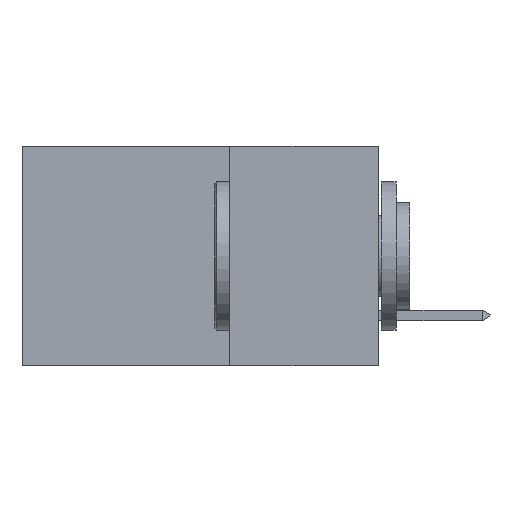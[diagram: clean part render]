
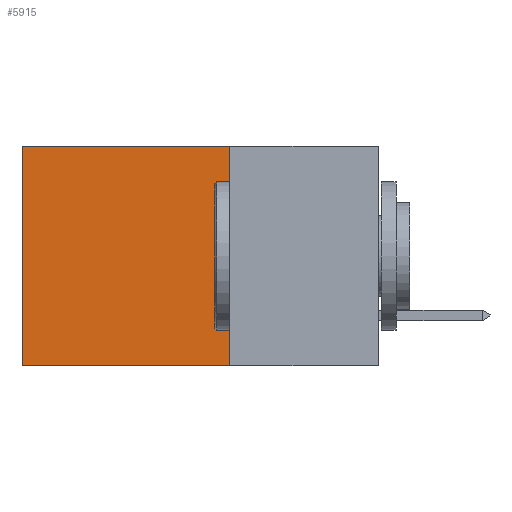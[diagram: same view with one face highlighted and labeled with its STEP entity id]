
A CAD part, left-side view. The second image highlights one B-rep face of the part: STEP entity #5915.
In plain terms, the highlighted planar face has unit normal (-1, 0, 0).
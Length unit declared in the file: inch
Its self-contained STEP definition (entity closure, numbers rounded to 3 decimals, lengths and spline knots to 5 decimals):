
#554 = VERTEX_POINT ( 'NONE', #1012 ) ;
#1012 = CARTESIAN_POINT ( 'NONE',  ( 0.2615, 0.25, -0.37 ) ) ;
#1763 = VERTEX_POINT ( 'NONE', #17823 ) ;
#1865 = EDGE_CURVE ( 'NONE', #14438, #1763, #7289, .T. ) ;
#3894 = CARTESIAN_POINT ( 'NONE',  ( 0.2615, 0.25, 0. ) ) ;
#4946 = CARTESIAN_POINT ( 'NONE',  ( 0.2615, 0.25, -0.37 ) ) ;
#5407 = ORIENTED_EDGE ( 'NONE', *, *, #11227, .F. ) ;
#5505 = CARTESIAN_POINT ( 'NONE',  ( 0.2615, 0.25, -0.37 ) ) ;
#5662 = DIRECTION ( 'NONE',  ( 0., 1., 0. ) ) ;
#5915 = ADVANCED_FACE ( 'NONE', ( #6634 ), #19309, .F. ) ;
#6634 = FACE_OUTER_BOUND ( 'NONE', #19253, .T. ) ;
#7289 = LINE ( 'NONE', #8921, #13518 ) ;
#8307 = VECTOR ( 'NONE', #5662, 39.37008 ) ;
#8531 = DIRECTION ( 'NONE',  ( 0., 1., 0. ) ) ;
#8921 = CARTESIAN_POINT ( 'NONE',  ( 0.2615, 0.25, 0. ) ) ;
#9086 = VECTOR ( 'NONE', #12416, 39.37008 ) ;
#9994 = LINE ( 'NONE', #11817, #8307 ) ;
#10129 = DIRECTION ( 'NONE',  ( 0., 0., -1. ) ) ;
#10196 = VERTEX_POINT ( 'NONE', #11056 ) ;
#10263 = AXIS2_PLACEMENT_3D ( 'NONE', #5505, #12889, #10129 ) ;
#10609 = VECTOR ( 'NONE', #11116, 39.37008 ) ;
#10910 = EDGE_CURVE ( 'NONE', #554, #10196, #9994, .T. ) ;
#11056 = CARTESIAN_POINT ( 'NONE',  ( 0.2615, 0.6, -0.37 ) ) ;
#11092 = CARTESIAN_POINT ( 'NONE',  ( 0.2615, 0.6, -0.37 ) ) ;
#11116 = DIRECTION ( 'NONE',  ( 0., 0., -1. ) ) ;
#11227 = EDGE_CURVE ( 'NONE', #14438, #554, #18964, .T. ) ;
#11817 = CARTESIAN_POINT ( 'NONE',  ( 0.2615, 0.25, -0.37 ) ) ;
#12039 = ORIENTED_EDGE ( 'NONE', *, *, #10910, .F. ) ;
#12416 = DIRECTION ( 'NONE',  ( 0., 0., -1. ) ) ;
#12889 = DIRECTION ( 'NONE',  ( 1., 0., 0. ) ) ;
#13518 = VECTOR ( 'NONE', #8531, 39.37008 ) ;
#13657 = ORIENTED_EDGE ( 'NONE', *, *, #1865, .T. ) ;
#14438 = VERTEX_POINT ( 'NONE', #3894 ) ;
#15531 = ORIENTED_EDGE ( 'NONE', *, *, #17687, .T. ) ;
#17188 = LINE ( 'NONE', #11092, #9086 ) ;
#17687 = EDGE_CURVE ( 'NONE', #1763, #10196, #17188, .T. ) ;
#17823 = CARTESIAN_POINT ( 'NONE',  ( 0.2615, 0.6, 0. ) ) ;
#18964 = LINE ( 'NONE', #4946, #10609 ) ;
#19253 = EDGE_LOOP ( 'NONE', ( #15531, #12039, #5407, #13657 ) ) ;
#19309 = PLANE ( 'NONE',  #10263 ) ;
